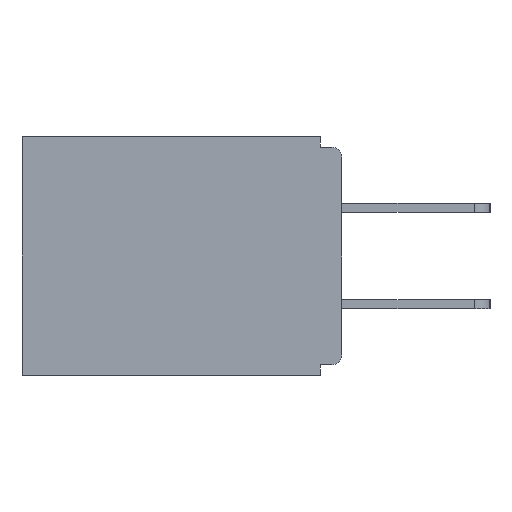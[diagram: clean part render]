
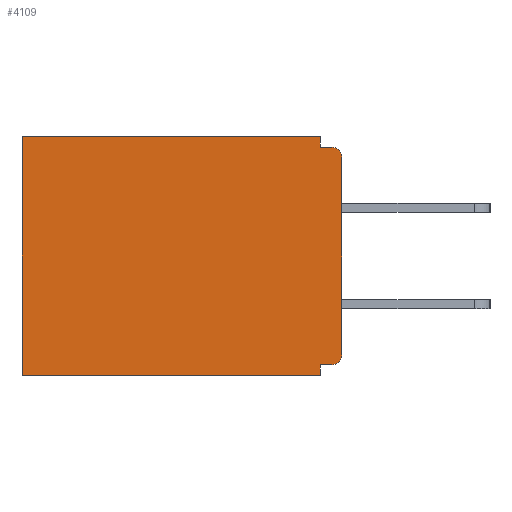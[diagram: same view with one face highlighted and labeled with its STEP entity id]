
A CAD part, left-side view. The second image highlights one B-rep face of the part: STEP entity #4109.
In plain terms, the highlighted planar face has unit normal (-1, 0, 0).
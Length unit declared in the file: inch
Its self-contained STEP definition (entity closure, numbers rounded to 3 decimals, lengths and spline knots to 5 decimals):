
#355 = CARTESIAN_POINT ( 'NONE',  ( 0.298, 0.031, -0.015 ) ) ;
#362 = CARTESIAN_POINT ( 'NONE',  ( 0.298, 0., -0.015 ) ) ;
#444 = EDGE_CURVE ( 'NONE', #11248, #2806, #8514, .T. ) ;
#460 = VERTEX_POINT ( 'NONE', #9429 ) ;
#1129 = LINE ( 'NONE', #362, #19401 ) ;
#1483 = EDGE_CURVE ( 'NONE', #22624, #460, #22574, .T. ) ;
#1889 = ORIENTED_EDGE ( 'NONE', *, *, #8437, .F. ) ;
#2071 = VERTEX_POINT ( 'NONE', #2632 ) ;
#2252 = EDGE_LOOP ( 'NONE', ( #6620, #17120, #17730, #17502, #19000, #4251, #5321, #15267, #9908, #1889 ) ) ;
#2277 = CARTESIAN_POINT ( 'NONE',  ( 0.298, 0.015, -0.328 ) ) ;
#2286 = LINE ( 'NONE', #21300, #2573 ) ;
#2573 = VECTOR ( 'NONE', #12561, 39.37008 ) ;
#2579 = CARTESIAN_POINT ( 'NONE',  ( 0.298, 0.031, 0. ) ) ;
#2632 = CARTESIAN_POINT ( 'NONE',  ( 0.298, 0.031, -0.343 ) ) ;
#2806 = VERTEX_POINT ( 'NONE', #355 ) ;
#3684 = DIRECTION ( 'NONE',  ( 0., -1., 0. ) ) ;
#3927 = CIRCLE ( 'NONE', #20385, 0.015 ) ;
#4109 = ADVANCED_FACE ( 'NONE', ( #14223 ), #16262, .F. ) ;
#4134 = VERTEX_POINT ( 'NONE', #18184 ) ;
#4251 = ORIENTED_EDGE ( 'NONE', *, *, #14769, .F. ) ;
#4730 = VERTEX_POINT ( 'NONE', #14277 ) ;
#4990 = LINE ( 'NONE', #11443, #22762 ) ;
#5321 = ORIENTED_EDGE ( 'NONE', *, *, #14547, .F. ) ;
#5467 = LINE ( 'NONE', #6449, #20974 ) ;
#6385 = CARTESIAN_POINT ( 'NONE',  ( 0.298, 0., -0.328 ) ) ;
#6449 = CARTESIAN_POINT ( 'NONE',  ( 0.298, 0., 0. ) ) ;
#6620 = ORIENTED_EDGE ( 'NONE', *, *, #17463, .T. ) ;
#7442 = CARTESIAN_POINT ( 'NONE',  ( 0.298, 0., 0. ) ) ;
#7517 = AXIS2_PLACEMENT_3D ( 'NONE', #7442, #19695, #14347 ) ;
#7813 = CARTESIAN_POINT ( 'NONE',  ( 0.298, 0., 0. ) ) ;
#8364 = CARTESIAN_POINT ( 'NONE',  ( 0.298, 0.46, -0.343 ) ) ;
#8437 = EDGE_CURVE ( 'NONE', #9863, #4730, #10233, .T. ) ;
#8514 = LINE ( 'NONE', #18313, #12673 ) ;
#9199 = DIRECTION ( 'NONE',  ( 0., 0., -1. ) ) ;
#9429 = CARTESIAN_POINT ( 'NONE',  ( 0.298, 0.031, -0.328 ) ) ;
#9726 = DIRECTION ( 'NONE',  ( 0., 0., -1. ) ) ;
#9863 = VERTEX_POINT ( 'NONE', #18543 ) ;
#9887 = CARTESIAN_POINT ( 'NONE',  ( 0.298, 0.46, 0. ) ) ;
#9908 = ORIENTED_EDGE ( 'NONE', *, *, #20580, .T. ) ;
#9939 = VERTEX_POINT ( 'NONE', #9887 ) ;
#10233 = LINE ( 'NONE', #7813, #19352 ) ;
#10519 = CARTESIAN_POINT ( 'NONE',  ( 0.298, 0.015, -0.03 ) ) ;
#11248 = VERTEX_POINT ( 'NONE', #2579 ) ;
#11436 = CIRCLE ( 'NONE', #12428, 0.015 ) ;
#11443 = CARTESIAN_POINT ( 'NONE',  ( 0.298, 0.46, 0. ) ) ;
#11573 = DIRECTION ( 'NONE',  ( 0., 1., 0. ) ) ;
#12097 = EDGE_CURVE ( 'NONE', #2806, #4134, #1129, .T. ) ;
#12235 = DIRECTION ( 'NONE',  ( 0., 0., -1. ) ) ;
#12428 = AXIS2_PLACEMENT_3D ( 'NONE', #15306, #13610, #19334 ) ;
#12561 = DIRECTION ( 'NONE',  ( 0., 0., -1. ) ) ;
#12673 = VECTOR ( 'NONE', #9199, 39.37008 ) ;
#13610 = DIRECTION ( 'NONE',  ( -1., 0., 0. ) ) ;
#14223 = FACE_OUTER_BOUND ( 'NONE', #2252, .T. ) ;
#14277 = CARTESIAN_POINT ( 'NONE',  ( 0.298, 0., -0.313 ) ) ;
#14347 = DIRECTION ( 'NONE',  ( 0., 0., -1. ) ) ;
#14547 = EDGE_CURVE ( 'NONE', #460, #2071, #2286, .T. ) ;
#14760 = LINE ( 'NONE', #15147, #18626 ) ;
#14769 = EDGE_CURVE ( 'NONE', #2071, #15679, #14760, .T. ) ;
#15147 = CARTESIAN_POINT ( 'NONE',  ( 0.298, 0., -0.343 ) ) ;
#15233 = DIRECTION ( 'NONE',  ( 0., 1., 0. ) ) ;
#15267 = ORIENTED_EDGE ( 'NONE', *, *, #1483, .F. ) ;
#15306 = CARTESIAN_POINT ( 'NONE',  ( 0.298, 0.015, -0.313 ) ) ;
#15679 = VERTEX_POINT ( 'NONE', #8364 ) ;
#16262 = PLANE ( 'NONE',  #7517 ) ;
#16969 = VECTOR ( 'NONE', #22145, 39.37008 ) ;
#17120 = ORIENTED_EDGE ( 'NONE', *, *, #12097, .F. ) ;
#17463 = EDGE_CURVE ( 'NONE', #9863, #4134, #3927, .T. ) ;
#17502 = ORIENTED_EDGE ( 'NONE', *, *, #22845, .T. ) ;
#17730 = ORIENTED_EDGE ( 'NONE', *, *, #444, .F. ) ;
#18184 = CARTESIAN_POINT ( 'NONE',  ( 0.298, 0.015, -0.015 ) ) ;
#18237 = DIRECTION ( 'NONE',  ( 0., 0., -1. ) ) ;
#18313 = CARTESIAN_POINT ( 'NONE',  ( 0.298, 0.031, -0.343 ) ) ;
#18543 = CARTESIAN_POINT ( 'NONE',  ( 0.298, 0., -0.03 ) ) ;
#18626 = VECTOR ( 'NONE', #15233, 39.37008 ) ;
#19000 = ORIENTED_EDGE ( 'NONE', *, *, #21644, .T. ) ;
#19334 = DIRECTION ( 'NONE',  ( 0., 0., -1. ) ) ;
#19352 = VECTOR ( 'NONE', #18237, 39.37008 ) ;
#19401 = VECTOR ( 'NONE', #3684, 39.37008 ) ;
#19566 = DIRECTION ( 'NONE',  ( -1., 0., 0. ) ) ;
#19695 = DIRECTION ( 'NONE',  ( 1., 0., 0. ) ) ;
#20385 = AXIS2_PLACEMENT_3D ( 'NONE', #10519, #19566, #12235 ) ;
#20580 = EDGE_CURVE ( 'NONE', #22624, #4730, #11436, .T. ) ;
#20974 = VECTOR ( 'NONE', #11573, 39.37008 ) ;
#21300 = CARTESIAN_POINT ( 'NONE',  ( 0.298, 0.031, -0.343 ) ) ;
#21644 = EDGE_CURVE ( 'NONE', #9939, #15679, #4990, .T. ) ;
#22145 = DIRECTION ( 'NONE',  ( 0., 1., 0. ) ) ;
#22574 = LINE ( 'NONE', #6385, #16969 ) ;
#22624 = VERTEX_POINT ( 'NONE', #2277 ) ;
#22762 = VECTOR ( 'NONE', #9726, 39.37008 ) ;
#22845 = EDGE_CURVE ( 'NONE', #11248, #9939, #5467, .T. ) ;
